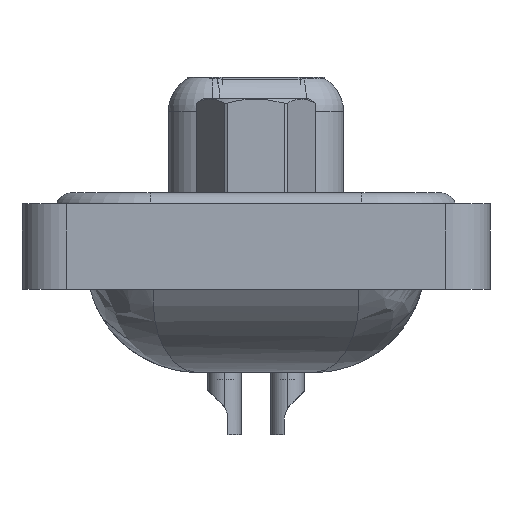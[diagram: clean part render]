
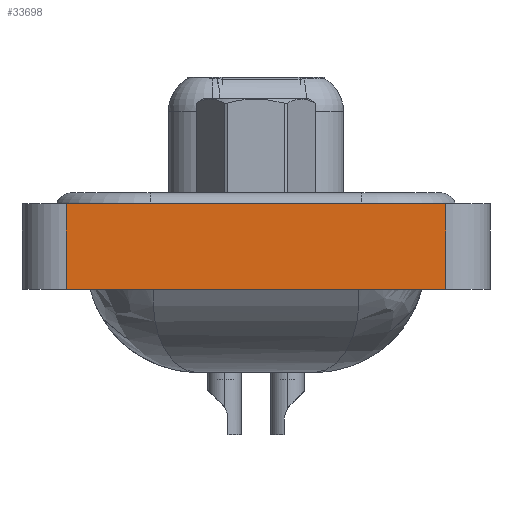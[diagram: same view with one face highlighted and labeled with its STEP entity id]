
A CAD part, left-side view. The second image highlights one B-rep face of the part: STEP entity #33698.
In plain terms, the highlighted planar face has unit normal (-1, 0, 0).
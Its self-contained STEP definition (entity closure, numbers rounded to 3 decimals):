
#1938 = FACE_OUTER_BOUND ( 'NONE', #32077, .T. ) ;
#2536 = CARTESIAN_POINT ( 'NONE',  ( -7.15, 8.55, 0.5 ) ) ;
#2857 = VERTEX_POINT ( 'NONE', #11628 ) ;
#6517 = VERTEX_POINT ( 'NONE', #2536 ) ;
#6525 = DIRECTION ( 'NONE',  ( -1., 0., 0. ) ) ;
#7403 = ORIENTED_EDGE ( 'NONE', *, *, #28131, .F. ) ;
#8477 = CARTESIAN_POINT ( 'NONE',  ( -7.15, -8.55, -3.35 ) ) ;
#8521 = VECTOR ( 'NONE', #13931, 1000. ) ;
#9620 = LINE ( 'NONE', #30941, #15039 ) ;
#11628 = CARTESIAN_POINT ( 'NONE',  ( -7.15, -8.55, 0.5 ) ) ;
#13726 = DIRECTION ( 'NONE',  ( 0., 0., 1. ) ) ;
#13931 = DIRECTION ( 'NONE',  ( 0., 0., 1. ) ) ;
#14079 = EDGE_CURVE ( 'NONE', #31566, #6517, #19346, .T. ) ;
#15009 = ORIENTED_EDGE ( 'NONE', *, *, #19692, .T. ) ;
#15039 = VECTOR ( 'NONE', #20362, 1000. ) ;
#15978 = VECTOR ( 'NONE', #25385, 1000. ) ;
#16374 = CARTESIAN_POINT ( 'NONE',  ( -7.15, -8.55, -3.35 ) ) ;
#17286 = DIRECTION ( 'NONE',  ( 0., 0., 1. ) ) ;
#18442 = CARTESIAN_POINT ( 'NONE',  ( -7.15, 8.55, -3.35 ) ) ;
#19346 = LINE ( 'NONE', #27105, #30344 ) ;
#19692 = EDGE_CURVE ( 'NONE', #31566, #29126, #34033, .T. ) ;
#19911 = CARTESIAN_POINT ( 'NONE',  ( -7.15, -8.55, -3.35 ) ) ;
#20362 = DIRECTION ( 'NONE',  ( 0., -1., 0. ) ) ;
#20637 = CARTESIAN_POINT ( 'NONE',  ( -7.15, -8.55, -3.35 ) ) ;
#22547 = PLANE ( 'NONE',  #24283 ) ;
#24283 = AXIS2_PLACEMENT_3D ( 'NONE', #19911, #6525, #17286 ) ;
#25385 = DIRECTION ( 'NONE',  ( 0., -1., 0. ) ) ;
#26020 = ORIENTED_EDGE ( 'NONE', *, *, #14079, .F. ) ;
#26446 = ORIENTED_EDGE ( 'NONE', *, *, #33509, .T. ) ;
#27105 = CARTESIAN_POINT ( 'NONE',  ( -7.15, 8.55, -3.35 ) ) ;
#28131 = EDGE_CURVE ( 'NONE', #6517, #2857, #9620, .T. ) ;
#29126 = VERTEX_POINT ( 'NONE', #16374 ) ;
#30344 = VECTOR ( 'NONE', #13726, 1000. ) ;
#30941 = CARTESIAN_POINT ( 'NONE',  ( -7.15, -8.55, 0.5 ) ) ;
#31566 = VERTEX_POINT ( 'NONE', #18442 ) ;
#32077 = EDGE_LOOP ( 'NONE', ( #26446, #7403, #26020, #15009 ) ) ;
#32611 = LINE ( 'NONE', #8477, #8521 ) ;
#33509 = EDGE_CURVE ( 'NONE', #29126, #2857, #32611, .T. ) ;
#33698 = ADVANCED_FACE ( 'NONE', ( #1938 ), #22547, .T. ) ;
#34033 = LINE ( 'NONE', #20637, #15978 ) ;
